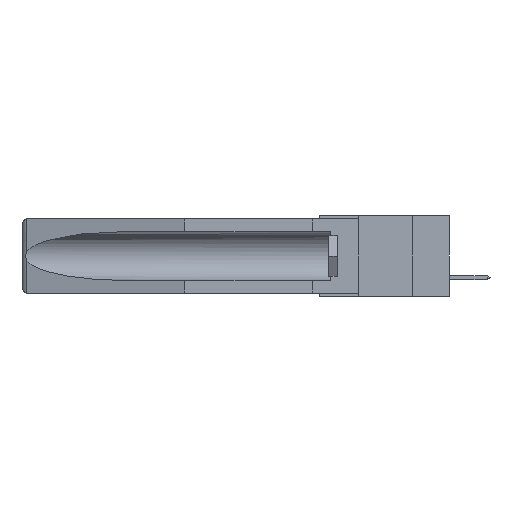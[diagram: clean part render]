
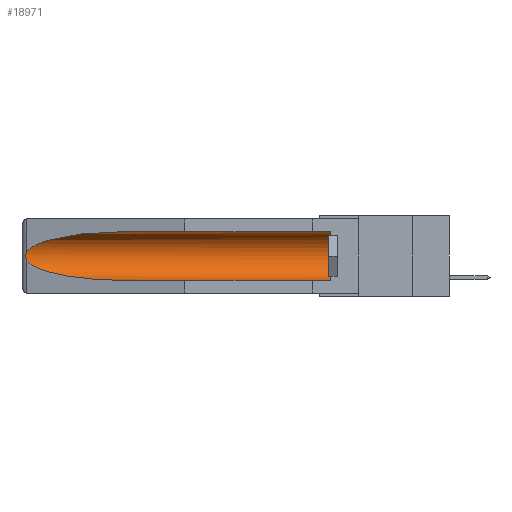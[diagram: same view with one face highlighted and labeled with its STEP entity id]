
A CAD part, left-side view. The second image highlights one B-rep face of the part: STEP entity #18971.
In plain terms, the highlighted cylindrical face has radius 2.857 mm (diameter 5.715 mm), a partial arc.
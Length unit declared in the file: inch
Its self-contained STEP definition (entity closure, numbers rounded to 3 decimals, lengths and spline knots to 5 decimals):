
#669 = VERTEX_POINT ( 'NONE', #10650 ) ;
#1550 = CIRCLE ( 'NONE', #12664, 0.1125 ) ;
#1630 = EDGE_CURVE ( 'NONE', #8877, #6297, #3283, .T. ) ;
#2493 = CARTESIAN_POINT ( 'NONE',  ( 0.2675, 1.53308, -0.16763 ) ) ;
#2622 = CARTESIAN_POINT ( 'NONE',  ( 0.26655, 1.53094, -0.18657 ) ) ;
#2863 = ORIENTED_EDGE ( 'NONE', *, *, #18551, .T. ) ;
#3207 = EDGE_CURVE ( 'NONE', #669, #12351, #17722, .T. ) ;
#3236 = FACE_OUTER_BOUND ( 'NONE', #7304, .T. ) ;
#3259 = DIRECTION ( 'NONE',  ( 0., 1., 0. ) ) ;
#3283 = B_SPLINE_CURVE_WITH_KNOTS ( 'NONE', 3,
 ( #5525, #5338, #17083, #11353, #2493, #3969, #17268, #2622, #17326, #8449 ),
 .UNSPECIFIED., .F., .F.,
 ( 4, 2, 2, 2, 4 ),
 ( 0., 0.00029, 0.00058, 0.00087, 0.00117 ),
 .UNSPECIFIED. ) ;
#3677 = CARTESIAN_POINT ( 'NONE',  ( 0.155, 0.126, -0.1715 ) ) ;
#3969 = CARTESIAN_POINT ( 'NONE',  ( 0.2675, 1.53308, -0.17534 ) ) ;
#4217 = EDGE_CURVE ( 'NONE', #8124, #8997, #15925, .T. ) ;
#5338 = CARTESIAN_POINT ( 'NONE',  ( 0.26597, 1.52961, -0.15275 ) ) ;
#5345 = ORIENTED_EDGE ( 'NONE', *, *, #3207, .F. ) ;
#5437 = CARTESIAN_POINT ( 'NONE',  ( 0.155, 0.126, -0.059 ) ) ;
#5456 = CARTESIAN_POINT ( 'NONE',  ( 0.26537, 1.52718, -0.14972 ) ) ;
#5525 = CARTESIAN_POINT ( 'NONE',  ( 0.26537, 1.52718, -0.14972 ) ) ;
#5609 = CARTESIAN_POINT ( 'NONE',  ( 0.155, -0.30754, -0.284 ) ) ;
#5782 = CARTESIAN_POINT ( 'NONE',  ( 0.155, 1.07973, -0.284 ) ) ;
#6012 = CYLINDRICAL_SURFACE ( 'NONE', #8472, 0.1125 ) ;
#6030 = CARTESIAN_POINT ( 'NONE',  ( 0.26537, 1.52718, -0.19328 ) ) ;
#6297 = VERTEX_POINT ( 'NONE', #6030 ) ;
#6667 = DIRECTION ( 'NONE',  ( 0., -1., 0. ) ) ;
#7111 = EDGE_CURVE ( 'NONE', #8997, #8877, #12997, .T. ) ;
#7304 = EDGE_LOOP ( 'NONE', ( #17896, #13802, #2863, #5345, #18934, #12802 ) ) ;
#8124 = VERTEX_POINT ( 'NONE', #5437 ) ;
#8449 = CARTESIAN_POINT ( 'NONE',  ( 0.26537, 1.52718, -0.19328 ) ) ;
#8472 = AXIS2_PLACEMENT_3D ( 'NONE', #8966, #3259, #15161 ) ;
#8877 = VERTEX_POINT ( 'NONE', #5456 ) ;
#8966 = CARTESIAN_POINT ( 'NONE',  ( 0.155, -0.30754, -0.1715 ) ) ;
#8997 = VERTEX_POINT ( 'NONE', #9709 ) ;
#9410 = CARTESIAN_POINT ( 'NONE',  ( 0.26537, 1.52718, -0.14972 ) ) ;
#9467 = CARTESIAN_POINT ( 'NONE',  ( 0.21114, 1.30732, -0.059 ) ) ;
#9709 = CARTESIAN_POINT ( 'NONE',  ( 0.155, 1.07973, -0.059 ) ) ;
#9784 = DIRECTION ( 'NONE',  ( 0., 1., 0. ) ) ;
#9909 = CARTESIAN_POINT ( 'NONE',  ( 0.155, -0.30754, -0.059 ) ) ;
#10650 = CARTESIAN_POINT ( 'NONE',  ( 0.155, 0.126, -0.284 ) ) ;
#10771 =( BOUNDED_CURVE ( )  B_SPLINE_CURVE ( 3, ( #11667, #14637, #19169, #5782 ),
 .UNSPECIFIED., .F., .T. ) 
 B_SPLINE_CURVE_WITH_KNOTS ( ( 4, 4 ),
 ( 0.1948, 1.5708 ),
 .UNSPECIFIED. ) 
 CURVE ( )  GEOMETRIC_REPRESENTATION_ITEM ( )  RATIONAL_B_SPLINE_CURVE ( ( 1., 0.848, 0.848, 1. ) ) 
 REPRESENTATION_ITEM ( '' )  );
#11353 = CARTESIAN_POINT ( 'NONE',  ( 0.2673, 1.5327, -0.16383 ) ) ;
#11667 = CARTESIAN_POINT ( 'NONE',  ( 0.26537, 1.52718, -0.19328 ) ) ;
#12351 = VERTEX_POINT ( 'NONE', #13687 ) ;
#12664 = AXIS2_PLACEMENT_3D ( 'NONE', #3677, #6667, #15491 ) ;
#12802 = ORIENTED_EDGE ( 'NONE', *, *, #4217, .T. ) ;
#12997 =( BOUNDED_CURVE ( )  B_SPLINE_CURVE ( 3, ( #14037, #9467, #15506, #9410 ),
 .UNSPECIFIED., .F., .F. ) 
 B_SPLINE_CURVE_WITH_KNOTS ( ( 4, 4 ),
 ( 4.71239, 6.08839 ),
 .UNSPECIFIED. ) 
 CURVE ( )  GEOMETRIC_REPRESENTATION_ITEM ( )  RATIONAL_B_SPLINE_CURVE ( ( 1., 0.848, 0.848, 1. ) ) 
 REPRESENTATION_ITEM ( '' )  );
#13687 = CARTESIAN_POINT ( 'NONE',  ( 0.155, 1.07973, -0.284 ) ) ;
#13802 = ORIENTED_EDGE ( 'NONE', *, *, #1630, .T. ) ;
#13811 = VECTOR ( 'NONE', #15991, 39.37008 ) ;
#14037 = CARTESIAN_POINT ( 'NONE',  ( 0.155, 1.07973, -0.059 ) ) ;
#14637 = CARTESIAN_POINT ( 'NONE',  ( 0.25451, 1.48313, -0.24835 ) ) ;
#15161 = DIRECTION ( 'NONE',  ( 0., 0., 1. ) ) ;
#15491 = DIRECTION ( 'NONE',  ( 0., 0., 1. ) ) ;
#15506 = CARTESIAN_POINT ( 'NONE',  ( 0.25451, 1.48313, -0.09465 ) ) ;
#15925 = LINE ( 'NONE', #9909, #18237 ) ;
#15991 = DIRECTION ( 'NONE',  ( 0., 1., 0. ) ) ;
#16390 = EDGE_CURVE ( 'NONE', #669, #8124, #1550, .T. ) ;
#17083 = CARTESIAN_POINT ( 'NONE',  ( 0.26654, 1.53092, -0.15636 ) ) ;
#17268 = CARTESIAN_POINT ( 'NONE',  ( 0.2673, 1.53269, -0.17917 ) ) ;
#17326 = CARTESIAN_POINT ( 'NONE',  ( 0.26597, 1.5296, -0.19026 ) ) ;
#17722 = LINE ( 'NONE', #5609, #13811 ) ;
#17896 = ORIENTED_EDGE ( 'NONE', *, *, #7111, .T. ) ;
#18237 = VECTOR ( 'NONE', #9784, 39.37008 ) ;
#18551 = EDGE_CURVE ( 'NONE', #6297, #12351, #10771, .T. ) ;
#18934 = ORIENTED_EDGE ( 'NONE', *, *, #16390, .T. ) ;
#18971 = ADVANCED_FACE ( 'NONE', ( #3236 ), #6012, .F. ) ;
#19169 = CARTESIAN_POINT ( 'NONE',  ( 0.21114, 1.30732, -0.284 ) ) ;
